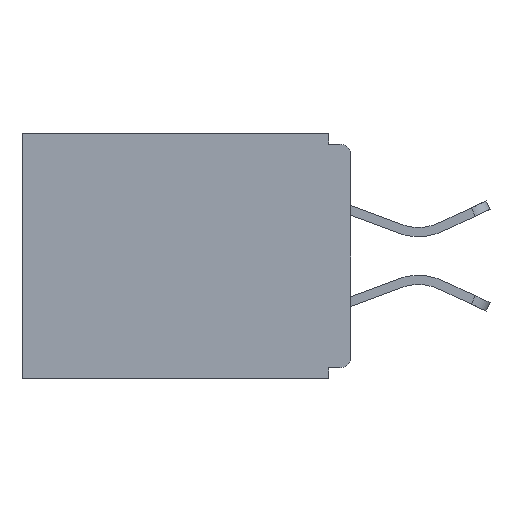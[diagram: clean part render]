
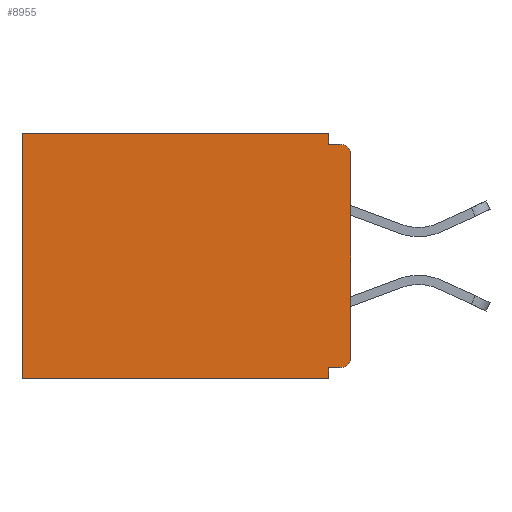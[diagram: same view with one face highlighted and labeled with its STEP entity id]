
A CAD part, left-side view. The second image highlights one B-rep face of the part: STEP entity #8955.
In plain terms, the highlighted planar face has unit normal (-1, 0, 0).
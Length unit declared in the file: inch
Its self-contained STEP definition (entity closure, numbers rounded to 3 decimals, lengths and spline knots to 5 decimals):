
#35 = CARTESIAN_POINT ( 'NONE',  ( 0.298, 0., -0.03 ) ) ;
#64 = LINE ( 'NONE', #13992, #4437 ) ;
#270 = LINE ( 'NONE', #10163, #14220 ) ;
#465 = CARTESIAN_POINT ( 'NONE',  ( 0.298, 0.031, -0.343 ) ) ;
#804 = VERTEX_POINT ( 'NONE', #35 ) ;
#888 = ORIENTED_EDGE ( 'NONE', *, *, #9612, .T. ) ;
#1222 = DIRECTION ( 'NONE',  ( 1., 0., 0. ) ) ;
#1422 = DIRECTION ( 'NONE',  ( -1., 0., 0. ) ) ;
#1429 = EDGE_LOOP ( 'NONE', ( #10981, #14428, #10063, #5539, #7889, #15125, #14203, #14238, #888, #10073 ) ) ;
#1789 = EDGE_CURVE ( 'NONE', #13440, #11802, #5826, .T. ) ;
#2148 = VERTEX_POINT ( 'NONE', #7823 ) ;
#2318 = CARTESIAN_POINT ( 'NONE',  ( 0.298, 0., 0. ) ) ;
#2635 = VECTOR ( 'NONE', #8753, 39.37008 ) ;
#3158 = EDGE_CURVE ( 'NONE', #14349, #2148, #6340, .T. ) ;
#3406 = EDGE_CURVE ( 'NONE', #11802, #5288, #64, .T. ) ;
#3820 = DIRECTION ( 'NONE',  ( 0., 0., -1. ) ) ;
#4014 = DIRECTION ( 'NONE',  ( 0., 0., -1. ) ) ;
#4437 = VECTOR ( 'NONE', #4524, 39.37008 ) ;
#4489 = EDGE_CURVE ( 'NONE', #804, #13577, #4580, .T. ) ;
#4524 = DIRECTION ( 'NONE',  ( 0., 1., 0. ) ) ;
#4580 = CIRCLE ( 'NONE', #12487, 0.015 ) ;
#4674 = AXIS2_PLACEMENT_3D ( 'NONE', #8670, #1422, #14567 ) ;
#4714 = CARTESIAN_POINT ( 'NONE',  ( 0.298, 0., -0.015 ) ) ;
#4767 = PLANE ( 'NONE',  #8284 ) ;
#5288 = VERTEX_POINT ( 'NONE', #11703 ) ;
#5539 = ORIENTED_EDGE ( 'NONE', *, *, #3158, .T. ) ;
#5760 = CARTESIAN_POINT ( 'NONE',  ( 0.298, 0., -0.313 ) ) ;
#5809 = CARTESIAN_POINT ( 'NONE',  ( 0.298, 0.031, -0.343 ) ) ;
#5826 = LINE ( 'NONE', #465, #2635 ) ;
#6035 = DIRECTION ( 'NONE',  ( -1., 0., 0. ) ) ;
#6232 = EDGE_CURVE ( 'NONE', #2148, #5288, #10758, .T. ) ;
#6340 = LINE ( 'NONE', #11505, #7056 ) ;
#6391 = CARTESIAN_POINT ( 'NONE',  ( 0.298, 0.031, -0.328 ) ) ;
#6638 = DIRECTION ( 'NONE',  ( 0., 0., -1. ) ) ;
#7056 = VECTOR ( 'NONE', #12034, 39.37008 ) ;
#7152 = VERTEX_POINT ( 'NONE', #5760 ) ;
#7220 = CARTESIAN_POINT ( 'NONE',  ( 0.298, 0.031, 0. ) ) ;
#7572 = CARTESIAN_POINT ( 'NONE',  ( 0.298, 0.46, 0. ) ) ;
#7604 = CARTESIAN_POINT ( 'NONE',  ( 0.298, 0.015, -0.03 ) ) ;
#7791 = LINE ( 'NONE', #2318, #15149 ) ;
#7796 = EDGE_CURVE ( 'NONE', #11164, #13440, #12832, .T. ) ;
#7823 = CARTESIAN_POINT ( 'NONE',  ( 0.298, 0.46, 0. ) ) ;
#7889 = ORIENTED_EDGE ( 'NONE', *, *, #6232, .T. ) ;
#8284 = AXIS2_PLACEMENT_3D ( 'NONE', #10897, #1222, #4014 ) ;
#8473 = CIRCLE ( 'NONE', #4674, 0.015 ) ;
#8670 = CARTESIAN_POINT ( 'NONE',  ( 0.298, 0.015, -0.313 ) ) ;
#8753 = DIRECTION ( 'NONE',  ( 0., 0., -1. ) ) ;
#8865 = VECTOR ( 'NONE', #3820, 39.37008 ) ;
#8955 = ADVANCED_FACE ( 'NONE', ( #12425 ), #4767, .F. ) ;
#9361 = DIRECTION ( 'NONE',  ( 0., 0., -1. ) ) ;
#9612 = EDGE_CURVE ( 'NONE', #11164, #7152, #8473, .T. ) ;
#9636 = VECTOR ( 'NONE', #11081, 39.37008 ) ;
#9893 = CARTESIAN_POINT ( 'NONE',  ( 0.298, 0., -0.328 ) ) ;
#10063 = ORIENTED_EDGE ( 'NONE', *, *, #15159, .F. ) ;
#10073 = ORIENTED_EDGE ( 'NONE', *, *, #12811, .F. ) ;
#10163 = CARTESIAN_POINT ( 'NONE',  ( 0.298, 0.031, -0.343 ) ) ;
#10520 = CARTESIAN_POINT ( 'NONE',  ( 0.298, 0.031, -0.015 ) ) ;
#10758 = LINE ( 'NONE', #7572, #8865 ) ;
#10785 = VECTOR ( 'NONE', #12129, 39.37008 ) ;
#10897 = CARTESIAN_POINT ( 'NONE',  ( 0.298, 0., 0. ) ) ;
#10981 = ORIENTED_EDGE ( 'NONE', *, *, #4489, .T. ) ;
#11081 = DIRECTION ( 'NONE',  ( 0., 1., 0. ) ) ;
#11164 = VERTEX_POINT ( 'NONE', #12880 ) ;
#11284 = CARTESIAN_POINT ( 'NONE',  ( 0.298, 0.015, -0.015 ) ) ;
#11505 = CARTESIAN_POINT ( 'NONE',  ( 0.298, 0., 0. ) ) ;
#11703 = CARTESIAN_POINT ( 'NONE',  ( 0.298, 0.46, -0.343 ) ) ;
#11802 = VERTEX_POINT ( 'NONE', #5809 ) ;
#11914 = LINE ( 'NONE', #4714, #10785 ) ;
#12034 = DIRECTION ( 'NONE',  ( 0., 1., 0. ) ) ;
#12129 = DIRECTION ( 'NONE',  ( 0., -1., 0. ) ) ;
#12425 = FACE_OUTER_BOUND ( 'NONE', #1429, .T. ) ;
#12487 = AXIS2_PLACEMENT_3D ( 'NONE', #7604, #6035, #13375 ) ;
#12811 = EDGE_CURVE ( 'NONE', #804, #7152, #7791, .T. ) ;
#12832 = LINE ( 'NONE', #9893, #9636 ) ;
#12880 = CARTESIAN_POINT ( 'NONE',  ( 0.298, 0.015, -0.328 ) ) ;
#13188 = EDGE_CURVE ( 'NONE', #15292, #13577, #11914, .T. ) ;
#13375 = DIRECTION ( 'NONE',  ( 0., 0., -1. ) ) ;
#13440 = VERTEX_POINT ( 'NONE', #6391 ) ;
#13577 = VERTEX_POINT ( 'NONE', #11284 ) ;
#13992 = CARTESIAN_POINT ( 'NONE',  ( 0.298, 0., -0.343 ) ) ;
#14203 = ORIENTED_EDGE ( 'NONE', *, *, #1789, .F. ) ;
#14220 = VECTOR ( 'NONE', #6638, 39.37008 ) ;
#14238 = ORIENTED_EDGE ( 'NONE', *, *, #7796, .F. ) ;
#14349 = VERTEX_POINT ( 'NONE', #7220 ) ;
#14428 = ORIENTED_EDGE ( 'NONE', *, *, #13188, .F. ) ;
#14567 = DIRECTION ( 'NONE',  ( 0., 0., -1. ) ) ;
#15125 = ORIENTED_EDGE ( 'NONE', *, *, #3406, .F. ) ;
#15149 = VECTOR ( 'NONE', #9361, 39.37008 ) ;
#15159 = EDGE_CURVE ( 'NONE', #14349, #15292, #270, .T. ) ;
#15292 = VERTEX_POINT ( 'NONE', #10520 ) ;
